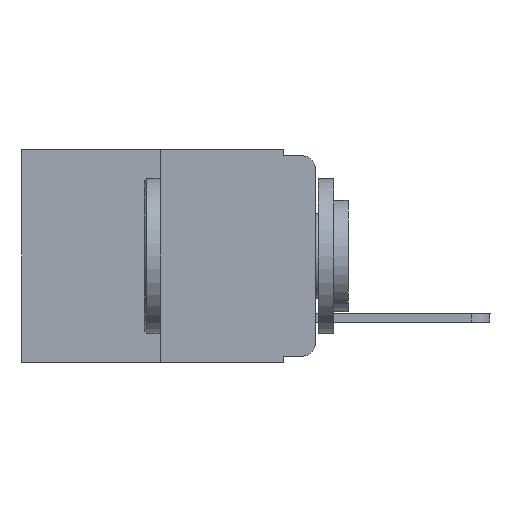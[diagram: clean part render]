
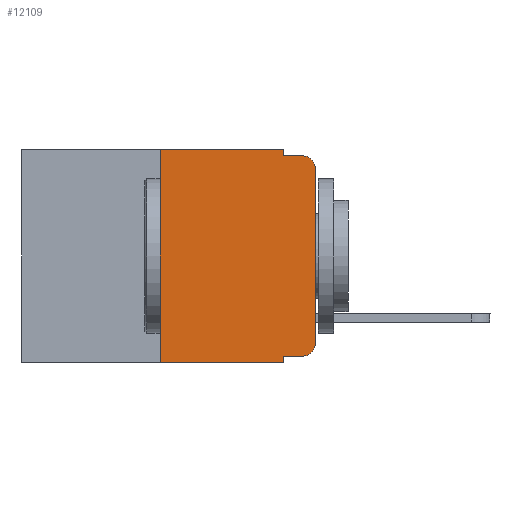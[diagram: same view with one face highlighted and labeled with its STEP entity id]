
A CAD part, left-side view. The second image highlights one B-rep face of the part: STEP entity #12109.
In plain terms, the highlighted planar face has unit normal (-1, 0, 0).
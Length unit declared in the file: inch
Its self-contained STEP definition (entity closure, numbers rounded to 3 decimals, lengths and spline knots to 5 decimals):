
#108 = DIRECTION ( 'NONE',  ( 0., 0., -1. ) ) ;
#380 = CARTESIAN_POINT ( 'NONE',  ( 0., 0.02, -0.03 ) ) ;
#432 = ORIENTED_EDGE ( 'NONE', *, *, #10483, .T. ) ;
#466 = ORIENTED_EDGE ( 'NONE', *, *, #6590, .T. ) ;
#525 = DIRECTION ( 'NONE',  ( 0., 0., -1. ) ) ;
#555 = VECTOR ( 'NONE', #8036, 39.37008 ) ;
#643 = CARTESIAN_POINT ( 'NONE',  ( 0., 0.051, -0.01 ) ) ;
#1072 = VECTOR ( 'NONE', #11465, 39.37008 ) ;
#1406 = LINE ( 'NONE', #11640, #4175 ) ;
#1427 = ORIENTED_EDGE ( 'NONE', *, *, #3022, .F. ) ;
#1444 = EDGE_CURVE ( 'NONE', #3836, #10743, #1406, .T. ) ;
#1465 = FACE_OUTER_BOUND ( 'NONE', #10988, .T. ) ;
#1615 = CARTESIAN_POINT ( 'NONE',  ( 0., 0.051, 0. ) ) ;
#1827 = EDGE_CURVE ( 'NONE', #7749, #3176, #6340, .T. ) ;
#2112 = ORIENTED_EDGE ( 'NONE', *, *, #2859, .T. ) ;
#2162 = PLANE ( 'NONE',  #8243 ) ;
#2483 = VERTEX_POINT ( 'NONE', #1615 ) ;
#2584 = DIRECTION ( 'NONE',  ( 0., 0., -1. ) ) ;
#2859 = EDGE_CURVE ( 'NONE', #4275, #8711, #9714, .T. ) ;
#3014 = ORIENTED_EDGE ( 'NONE', *, *, #3367, .F. ) ;
#3022 = EDGE_CURVE ( 'NONE', #2483, #11886, #4427, .T. ) ;
#3087 = VERTEX_POINT ( 'NONE', #10945 ) ;
#3176 = VERTEX_POINT ( 'NONE', #7361 ) ;
#3367 = EDGE_CURVE ( 'NONE', #3836, #3087, #10165, .T. ) ;
#3437 = DIRECTION ( 'NONE',  ( 0., -1., 0. ) ) ;
#3836 = VERTEX_POINT ( 'NONE', #7798 ) ;
#4121 = CIRCLE ( 'NONE', #10495, 0.02 ) ;
#4142 = CARTESIAN_POINT ( 'NONE',  ( 0., 0.25, -0.343 ) ) ;
#4156 = LINE ( 'NONE', #8773, #10592 ) ;
#4162 = VECTOR ( 'NONE', #6941, 39.37008 ) ;
#4175 = VECTOR ( 'NONE', #9844, 39.37008 ) ;
#4216 = LINE ( 'NONE', #10043, #555 ) ;
#4275 = VERTEX_POINT ( 'NONE', #11062 ) ;
#4280 = VECTOR ( 'NONE', #525, 39.37008 ) ;
#4427 = LINE ( 'NONE', #7120, #5010 ) ;
#4950 = CARTESIAN_POINT ( 'NONE',  ( 0., 0., 0. ) ) ;
#5010 = VECTOR ( 'NONE', #2584, 39.37008 ) ;
#5320 = DIRECTION ( 'NONE',  ( 0., 0., -1. ) ) ;
#5590 = CARTESIAN_POINT ( 'NONE',  ( 0., 0., -0.03 ) ) ;
#5704 = CARTESIAN_POINT ( 'NONE',  ( 0., 0.473, 0. ) ) ;
#5791 = AXIS2_PLACEMENT_3D ( 'NONE', #380, #7903, #9752 ) ;
#6340 = LINE ( 'NONE', #8768, #4162 ) ;
#6590 = EDGE_CURVE ( 'NONE', #7749, #3087, #4216, .T. ) ;
#6721 = DIRECTION ( 'NONE',  ( 1., 0., 0. ) ) ;
#6869 = DIRECTION ( 'NONE',  ( 0., -1., 0. ) ) ;
#6941 = DIRECTION ( 'NONE',  ( 0., 0., 1. ) ) ;
#7120 = CARTESIAN_POINT ( 'NONE',  ( 0., 0.051, 0. ) ) ;
#7361 = CARTESIAN_POINT ( 'NONE',  ( 0., 0.25, 0. ) ) ;
#7431 = ORIENTED_EDGE ( 'NONE', *, *, #10563, .F. ) ;
#7749 = VERTEX_POINT ( 'NONE', #4142 ) ;
#7798 = CARTESIAN_POINT ( 'NONE',  ( 0., 0.051, -0.333 ) ) ;
#7903 = DIRECTION ( 'NONE',  ( -1., 0., 0. ) ) ;
#7930 = CARTESIAN_POINT ( 'NONE',  ( 0., 0.051, 0. ) ) ;
#8036 = DIRECTION ( 'NONE',  ( 0., -1., 0. ) ) ;
#8080 = VECTOR ( 'NONE', #3437, 39.37008 ) ;
#8243 = AXIS2_PLACEMENT_3D ( 'NONE', #5704, #6721, #108 ) ;
#8293 = CARTESIAN_POINT ( 'NONE',  ( 0., 0.02, -0.333 ) ) ;
#8454 = ORIENTED_EDGE ( 'NONE', *, *, #1827, .F. ) ;
#8464 = VERTEX_POINT ( 'NONE', #9046 ) ;
#8711 = VERTEX_POINT ( 'NONE', #5590 ) ;
#8768 = CARTESIAN_POINT ( 'NONE',  ( 0., 0.25, 0. ) ) ;
#8773 = CARTESIAN_POINT ( 'NONE',  ( 0., 0.051, -0.01 ) ) ;
#8952 = CIRCLE ( 'NONE', #5791, 0.02 ) ;
#9026 = CARTESIAN_POINT ( 'NONE',  ( 0., 0.473, 0. ) ) ;
#9046 = CARTESIAN_POINT ( 'NONE',  ( 0., 0.02, -0.01 ) ) ;
#9078 = ORIENTED_EDGE ( 'NONE', *, *, #9407, .F. ) ;
#9334 = ORIENTED_EDGE ( 'NONE', *, *, #10991, .T. ) ;
#9407 = EDGE_CURVE ( 'NONE', #11886, #8464, #4156, .T. ) ;
#9714 = LINE ( 'NONE', #4950, #1072 ) ;
#9752 = DIRECTION ( 'NONE',  ( 0., 0., -1. ) ) ;
#9844 = DIRECTION ( 'NONE',  ( 0., -1., 0. ) ) ;
#10043 = CARTESIAN_POINT ( 'NONE',  ( 0., 0.473, -0.343 ) ) ;
#10165 = LINE ( 'NONE', #7930, #4280 ) ;
#10483 = EDGE_CURVE ( 'NONE', #10743, #4275, #4121, .T. ) ;
#10495 = AXIS2_PLACEMENT_3D ( 'NONE', #10848, #10931, #5320 ) ;
#10559 = LINE ( 'NONE', #9026, #8080 ) ;
#10563 = EDGE_CURVE ( 'NONE', #3176, #2483, #10559, .T. ) ;
#10592 = VECTOR ( 'NONE', #6869, 39.37008 ) ;
#10743 = VERTEX_POINT ( 'NONE', #8293 ) ;
#10848 = CARTESIAN_POINT ( 'NONE',  ( 0., 0.02, -0.313 ) ) ;
#10931 = DIRECTION ( 'NONE',  ( -1., 0., 0. ) ) ;
#10945 = CARTESIAN_POINT ( 'NONE',  ( 0., 0.051, -0.343 ) ) ;
#10988 = EDGE_LOOP ( 'NONE', ( #2112, #9334, #9078, #1427, #7431, #8454, #466, #3014, #11495, #432 ) ) ;
#10991 = EDGE_CURVE ( 'NONE', #8711, #8464, #8952, .T. ) ;
#11062 = CARTESIAN_POINT ( 'NONE',  ( 0., 0., -0.313 ) ) ;
#11465 = DIRECTION ( 'NONE',  ( 0., 0., 1. ) ) ;
#11495 = ORIENTED_EDGE ( 'NONE', *, *, #1444, .T. ) ;
#11640 = CARTESIAN_POINT ( 'NONE',  ( 0., 0.051, -0.333 ) ) ;
#11886 = VERTEX_POINT ( 'NONE', #643 ) ;
#12109 = ADVANCED_FACE ( 'NONE', ( #1465 ), #2162, .F. ) ;
